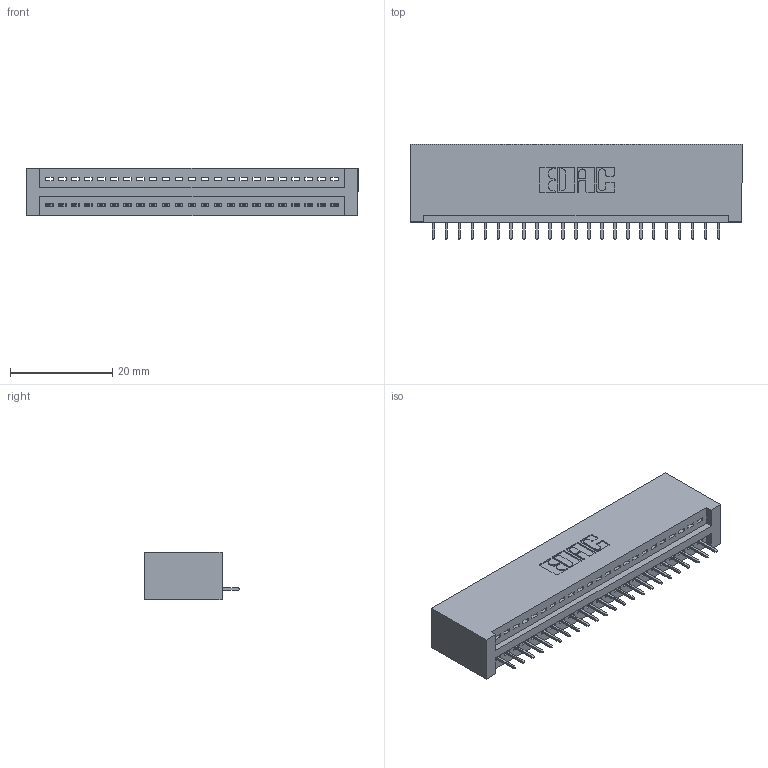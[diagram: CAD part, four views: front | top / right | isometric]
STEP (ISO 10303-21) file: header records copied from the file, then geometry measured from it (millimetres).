
FILE_DESCRIPTION (( 'STEP AP203' ), '1' );
FILE_NAME ('845-023-525-101.STEP', '2020-09-22T21:09:09', ( '' ), ( '' ), 'SwSTEP 2.0', 'SolidWorks 2020', '' );
FILE_SCHEMA (( 'CONFIG_CONTROL_DESIGN' ));
Length unit declared in the file: inch
Products named in the file (3): 845-023-525-101; 345-292-001_345-293-125; 845 Part_No Mounting Lugs
Assembly tree (24 placements, depth 2):
  845-023-525-101
    845 Part_No Mounting Lugs
    345-292-001_345-293-125  x23
Bounding box: 65.02 x 18.72 x 9.4 mm (x, y, z)
Volume: 6510.9 mm3; surface area: 8271.1 mm2
Topology: 24 solids, 24 shells, 1544 faces, 4457 edges, 2878 vertices
Faces by surface type: plane 1134, cylinder 410
Entity records: 19665 total; most frequent: CARTESIAN_POINT 3413, ORIENTED_EDGE 3370, DIRECTION 3003, EDGE_CURVE 1685, LINE 1473, VECTOR 1473, VERTEX_POINT 1118, AXIS2_PLACEMENT_3D 765
